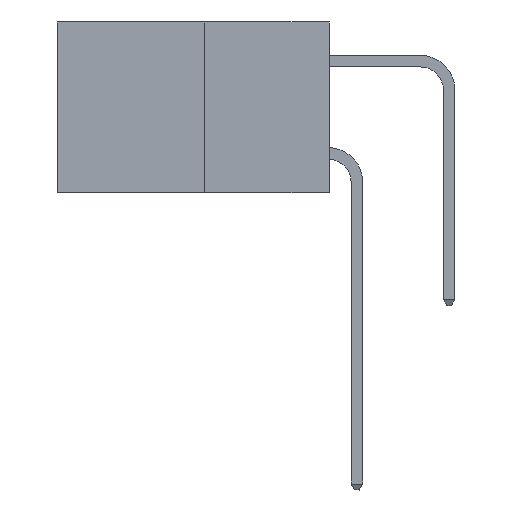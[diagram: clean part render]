
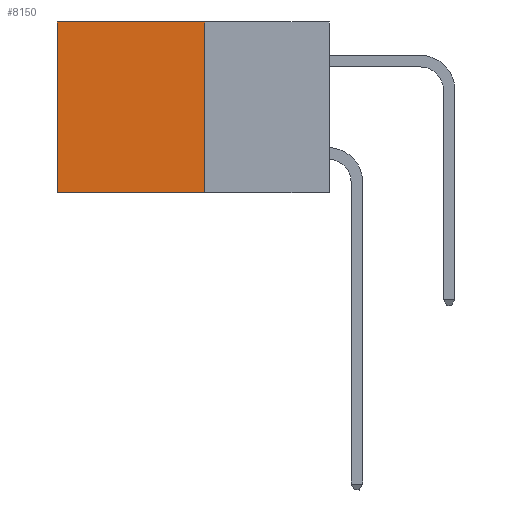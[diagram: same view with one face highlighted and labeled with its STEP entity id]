
A CAD part, left-side view. The second image highlights one B-rep face of the part: STEP entity #8150.
In plain terms, the highlighted planar face has unit normal (-1, 0, 0).
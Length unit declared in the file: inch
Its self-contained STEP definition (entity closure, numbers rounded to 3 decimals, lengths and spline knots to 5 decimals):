
#734 = CARTESIAN_POINT ( 'NONE',  ( 0.277, 0.27, -0.37 ) ) ;
#891 = EDGE_CURVE ( 'NONE', #6355, #5668, #15385, .T. ) ;
#1020 = CARTESIAN_POINT ( 'NONE',  ( 0.277, 0.27, -0.37 ) ) ;
#1302 = ORIENTED_EDGE ( 'NONE', *, *, #11642, .T. ) ;
#1494 = CARTESIAN_POINT ( 'NONE',  ( 0.277, 0.27, 0. ) ) ;
#1527 = DIRECTION ( 'NONE',  ( 0., 0., -1. ) ) ;
#2440 = DIRECTION ( 'NONE',  ( 0., 1., 0. ) ) ;
#4469 = CARTESIAN_POINT ( 'NONE',  ( 0.277, 0.59, -0.37 ) ) ;
#4597 = CARTESIAN_POINT ( 'NONE',  ( 0.277, 0.27, -0.37 ) ) ;
#5575 = DIRECTION ( 'NONE',  ( 1., 0., 0. ) ) ;
#5668 = VERTEX_POINT ( 'NONE', #18291 ) ;
#6355 = VERTEX_POINT ( 'NONE', #4597 ) ;
#6366 = ORIENTED_EDGE ( 'NONE', *, *, #9924, .T. ) ;
#7162 = VECTOR ( 'NONE', #2440, 39.37008 ) ;
#7467 = VECTOR ( 'NONE', #16306, 39.37008 ) ;
#7532 = EDGE_LOOP ( 'NONE', ( #6366, #7608, #12031, #1302 ) ) ;
#7533 = LINE ( 'NONE', #734, #14559 ) ;
#7608 = ORIENTED_EDGE ( 'NONE', *, *, #891, .F. ) ;
#7629 = VERTEX_POINT ( 'NONE', #1494 ) ;
#8150 = ADVANCED_FACE ( 'NONE', ( #16598 ), #14029, .F. ) ;
#8573 = CARTESIAN_POINT ( 'NONE',  ( 0.277, 0.27, -0.37 ) ) ;
#8708 = VERTEX_POINT ( 'NONE', #11975 ) ;
#9924 = EDGE_CURVE ( 'NONE', #8708, #5668, #18019, .T. ) ;
#10473 = LINE ( 'NONE', #11083, #7162 ) ;
#11083 = CARTESIAN_POINT ( 'NONE',  ( 0.277, 0.27, 0. ) ) ;
#11642 = EDGE_CURVE ( 'NONE', #7629, #8708, #10473, .T. ) ;
#11975 = CARTESIAN_POINT ( 'NONE',  ( 0.277, 0.59, 0. ) ) ;
#11987 = AXIS2_PLACEMENT_3D ( 'NONE', #1020, #5575, #15455 ) ;
#12031 = ORIENTED_EDGE ( 'NONE', *, *, #14095, .F. ) ;
#12285 = DIRECTION ( 'NONE',  ( 0., 0., -1. ) ) ;
#14029 = PLANE ( 'NONE',  #11987 ) ;
#14095 = EDGE_CURVE ( 'NONE', #7629, #6355, #7533, .T. ) ;
#14559 = VECTOR ( 'NONE', #12285, 39.37008 ) ;
#15385 = LINE ( 'NONE', #8573, #7467 ) ;
#15455 = DIRECTION ( 'NONE',  ( 0., 0., -1. ) ) ;
#16306 = DIRECTION ( 'NONE',  ( 0., 1., 0. ) ) ;
#16598 = FACE_OUTER_BOUND ( 'NONE', #7532, .T. ) ;
#17617 = VECTOR ( 'NONE', #1527, 39.37008 ) ;
#18019 = LINE ( 'NONE', #4469, #17617 ) ;
#18291 = CARTESIAN_POINT ( 'NONE',  ( 0.277, 0.59, -0.37 ) ) ;
